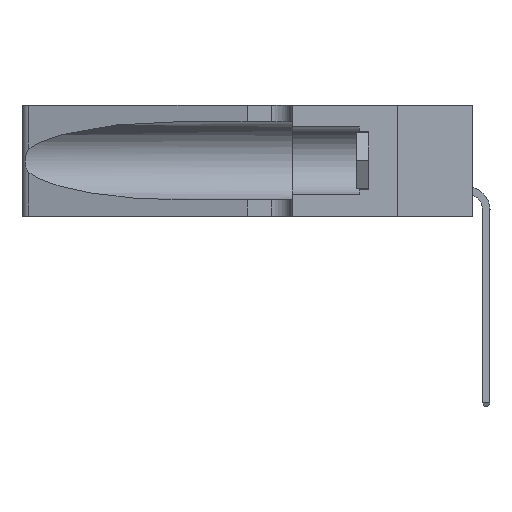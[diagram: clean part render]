
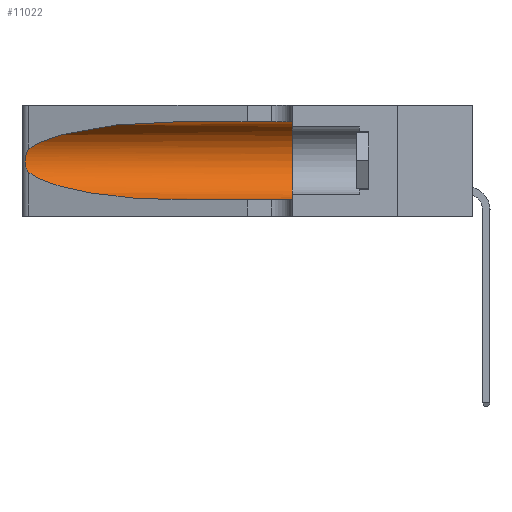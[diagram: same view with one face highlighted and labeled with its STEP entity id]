
A CAD part, left-side view. The second image highlights one B-rep face of the part: STEP entity #11022.
In plain terms, the highlighted cylindrical face has radius 3.308 mm (diameter 6.617 mm), a partial arc.
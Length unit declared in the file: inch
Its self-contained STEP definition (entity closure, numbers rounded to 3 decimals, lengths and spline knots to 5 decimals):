
#363 = EDGE_LOOP ( 'NONE', ( #15283, #25350, #43719, #14199, #26057, #25851 ) ) ;
#3106 = CARTESIAN_POINT ( 'NONE',  ( 0.2373, 1.15595, 0.08982 ) ) ;
#3523 = CARTESIAN_POINT ( 'NONE',  ( 0.25487, 1.22718, 0.14631 ) ) ;
#4345 = B_SPLINE_CURVE_WITH_KNOTS ( 'NONE', 3,
 ( #43695, #33019, #16075, #30004, #12313, #36508, #5440, #15775, #23076, #9120, #26543, #29686, #5739, #36362 ),
 .UNSPECIFIED., .F., .F.,
 ( 4, 2, 2, 2, 2, 2, 4 ),
 ( 0., 0.00027, 0.00053, 0.00107, 0.0016, 0.00187, 0.00214 ),
 .UNSPECIFIED. ) ;
#5391 = VERTEX_POINT ( 'NONE', #42539 ) ;
#5440 = CARTESIAN_POINT ( 'NONE',  ( 0.26075, 1.23896, 0.19203 ) ) ;
#5623 = AXIS2_PLACEMENT_3D ( 'NONE', #23888, #16481, #13317 ) ;
#5739 = CARTESIAN_POINT ( 'NONE',  ( 0.25555, 1.22993, 0.14849 ) ) ;
#6287 = LINE ( 'NONE', #29666, #23691 ) ;
#9120 = CARTESIAN_POINT ( 'NONE',  ( 0.25856, 1.23593, 0.16098 ) ) ;
#9895 = VERTEX_POINT ( 'NONE', #10203 ) ;
#10203 = CARTESIAN_POINT ( 'NONE',  ( 0.25487, 1.22718, 0.22369 ) ) ;
#11022 = ADVANCED_FACE ( 'NONE', ( #31299 ), #28041, .F. ) ;
#11990 = EDGE_CURVE ( 'NONE', #42610, #5391, #6287, .T. ) ;
#12313 = CARTESIAN_POINT ( 'NONE',  ( 0.25854, 1.2359, 0.20912 ) ) ;
#12923 = CARTESIAN_POINT ( 'NONE',  ( 0.25487, 1.22718, 0.22369 ) ) ;
#13110 = CARTESIAN_POINT ( 'NONE',  ( 0.1305, 0.72297, 0.31525 ) ) ;
#13181 = VERTEX_POINT ( 'NONE', #26400 ) ;
#13317 = DIRECTION ( 'NONE',  ( 0., 0., -1. ) ) ;
#13364 = EDGE_CURVE ( 'NONE', #13181, #30204, #26809, .T. ) ;
#14199 = ORIENTED_EDGE ( 'NONE', *, *, #13364, .T. ) ;
#15126 = CIRCLE ( 'NONE', #19793, 0.13025 ) ;
#15283 = ORIENTED_EDGE ( 'NONE', *, *, #28581, .T. ) ;
#15768 = VERTEX_POINT ( 'NONE', #3523 ) ;
#15775 = CARTESIAN_POINT ( 'NONE',  ( 0.26075, 1.23896, 0.178 ) ) ;
#16075 = CARTESIAN_POINT ( 'NONE',  ( 0.25639, 1.23184, 0.21858 ) ) ;
#16481 = DIRECTION ( 'NONE',  ( 0., -1., 0. ) ) ;
#16690 =( BOUNDED_CURVE ( )  B_SPLINE_CURVE ( 3, ( #24209, #3106, #41219, #21011 ),
 .UNSPECIFIED., .F., .T. ) 
 B_SPLINE_CURVE_WITH_KNOTS ( ( 4, 4 ),
 ( 3.44316, 4.71239 ),
 .UNSPECIFIED. ) 
 CURVE ( )  GEOMETRIC_REPRESENTATION_ITEM ( )  RATIONAL_B_SPLINE_CURVE ( ( 1., 0.87, 0.87, 1. ) ) 
 REPRESENTATION_ITEM ( '' )  );
#17539 = CARTESIAN_POINT ( 'NONE',  ( 0.1305, 0.35, 0.185 ) ) ;
#19793 = AXIS2_PLACEMENT_3D ( 'NONE', #17539, #31177, #31447 ) ;
#20315 = CARTESIAN_POINT ( 'NONE',  ( 0.1305, 0.72297, 0.31525 ) ) ;
#21011 = CARTESIAN_POINT ( 'NONE',  ( 0.1305, 0.72297, 0.05475 ) ) ;
#21893 = EDGE_CURVE ( 'NONE', #15768, #13181, #16690, .T. ) ;
#23076 = CARTESIAN_POINT ( 'NONE',  ( 0.26017, 1.23833, 0.17102 ) ) ;
#23566 = DIRECTION ( 'NONE',  ( 0., -1., 0. ) ) ;
#23691 = VECTOR ( 'NONE', #36479, 39.37008 ) ;
#23888 = CARTESIAN_POINT ( 'NONE',  ( 0.1305, 1.61858, 0.185 ) ) ;
#24068 = CARTESIAN_POINT ( 'NONE',  ( 0.1305, 0.35, 0.05475 ) ) ;
#24209 = CARTESIAN_POINT ( 'NONE',  ( 0.25487, 1.22718, 0.14631 ) ) ;
#25350 = ORIENTED_EDGE ( 'NONE', *, *, #29244, .T. ) ;
#25851 = ORIENTED_EDGE ( 'NONE', *, *, #11990, .F. ) ;
#26057 = ORIENTED_EDGE ( 'NONE', *, *, #41292, .F. ) ;
#26400 = CARTESIAN_POINT ( 'NONE',  ( 0.1305, 0.72297, 0.05475 ) ) ;
#26543 = CARTESIAN_POINT ( 'NONE',  ( 0.25789, 1.23486, 0.15765 ) ) ;
#26729 = CARTESIAN_POINT ( 'NONE',  ( 0.1305, 1.61858, 0.05475 ) ) ;
#26809 = LINE ( 'NONE', #26729, #31593 ) ;
#26988 = CARTESIAN_POINT ( 'NONE',  ( 0.18966, 0.96281, 0.31525 ) ) ;
#28041 = CYLINDRICAL_SURFACE ( 'NONE', #5623, 0.13025 ) ;
#28581 = EDGE_CURVE ( 'NONE', #42610, #9895, #36088, .T. ) ;
#29244 = EDGE_CURVE ( 'NONE', #9895, #15768, #4345, .T. ) ;
#29666 = CARTESIAN_POINT ( 'NONE',  ( 0.1305, 1.61858, 0.31525 ) ) ;
#29686 = CARTESIAN_POINT ( 'NONE',  ( 0.25639, 1.23186, 0.15144 ) ) ;
#30004 = CARTESIAN_POINT ( 'NONE',  ( 0.25787, 1.23484, 0.2124 ) ) ;
#30204 = VERTEX_POINT ( 'NONE', #24068 ) ;
#31177 = DIRECTION ( 'NONE',  ( 0., 1., 0. ) ) ;
#31299 = FACE_OUTER_BOUND ( 'NONE', #363, .T. ) ;
#31447 = DIRECTION ( 'NONE',  ( 0., 0., 1. ) ) ;
#31593 = VECTOR ( 'NONE', #23566, 39.37008 ) ;
#33019 = CARTESIAN_POINT ( 'NONE',  ( 0.25555, 1.22994, 0.2215 ) ) ;
#36088 =( BOUNDED_CURVE ( )  B_SPLINE_CURVE ( 3, ( #20315, #26988, #41090, #12923 ),
 .UNSPECIFIED., .F., .F. ) 
 B_SPLINE_CURVE_WITH_KNOTS ( ( 4, 4 ),
 ( 1.5708, 2.84003 ),
 .UNSPECIFIED. ) 
 CURVE ( )  GEOMETRIC_REPRESENTATION_ITEM ( )  RATIONAL_B_SPLINE_CURVE ( ( 1., 0.87, 0.87, 1. ) ) 
 REPRESENTATION_ITEM ( '' )  );
#36362 = CARTESIAN_POINT ( 'NONE',  ( 0.25487, 1.22718, 0.14631 ) ) ;
#36479 = DIRECTION ( 'NONE',  ( 0., -1., 0. ) ) ;
#36508 = CARTESIAN_POINT ( 'NONE',  ( 0.26018, 1.23835, 0.19895 ) ) ;
#41090 = CARTESIAN_POINT ( 'NONE',  ( 0.2373, 1.15595, 0.28018 ) ) ;
#41219 = CARTESIAN_POINT ( 'NONE',  ( 0.18966, 0.96281, 0.05475 ) ) ;
#41292 = EDGE_CURVE ( 'NONE', #5391, #30204, #15126, .T. ) ;
#42539 = CARTESIAN_POINT ( 'NONE',  ( 0.1305, 0.35, 0.31525 ) ) ;
#42610 = VERTEX_POINT ( 'NONE', #13110 ) ;
#43695 = CARTESIAN_POINT ( 'NONE',  ( 0.25487, 1.22718, 0.22369 ) ) ;
#43719 = ORIENTED_EDGE ( 'NONE', *, *, #21893, .T. ) ;
